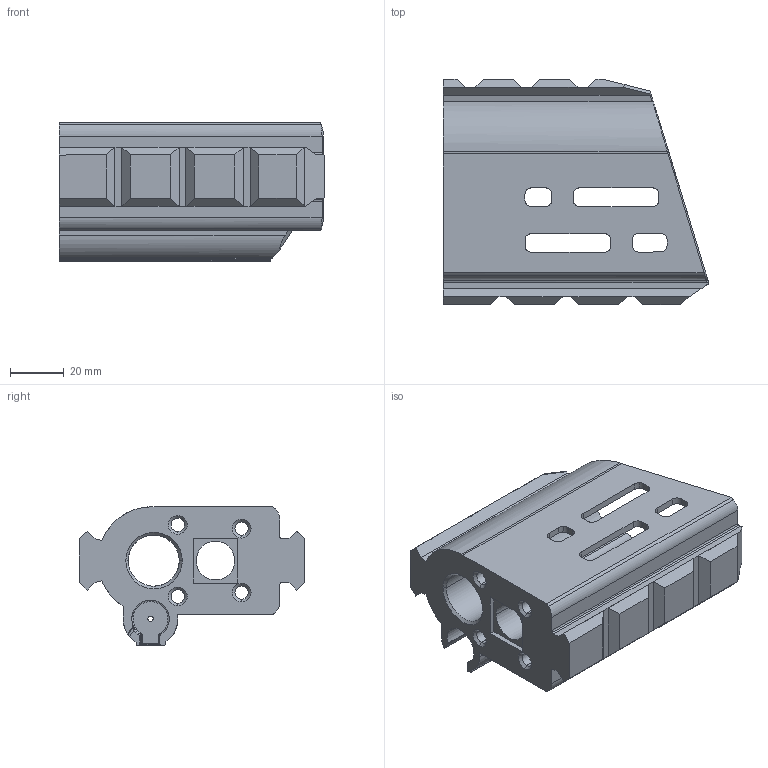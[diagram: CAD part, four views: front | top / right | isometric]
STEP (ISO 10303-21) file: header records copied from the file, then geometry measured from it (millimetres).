
FILE_DESCRIPTION(('STEP AP214'),'1');
FILE_NAME('Mlok barrel retainer.stp','2020-07-19T07:46:45',(' '),(' '),'Spatial InterOp 3D',' ',' ');
FILE_SCHEMA(('AUTOMOTIVE_DESIGN { 1 0 10303 214 1 1 1 1 }'));
Length unit declared in the file: metre
Products named in the file (1): ASM Body
Bounding box: 99.02 x 84.21 x 51.68 mm (x, y, z)
Volume: 129719.4 mm3; surface area: 43748.2 mm2
Topology: 1 solids, 1 shells, 288 faces, 836 edges, 541 vertices
Faces by surface type: plane 132, cylinder 128, cone 12, bspline 11, torus 4, sphere 1
Entity records: 11538 total; most frequent: CARTESIAN_POINT 3779, ORIENTED_EDGE 1668, DIRECTION 1601, EDGE_CURVE 834, AXIS2_PLACEMENT_3D 547, VERTEX_POINT 541, LINE 507, VECTOR 507
